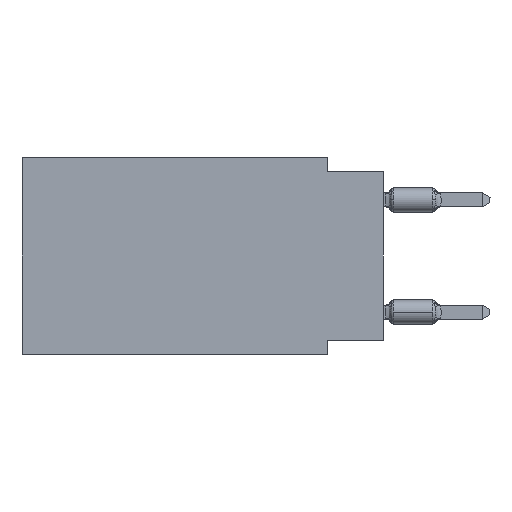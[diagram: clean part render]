
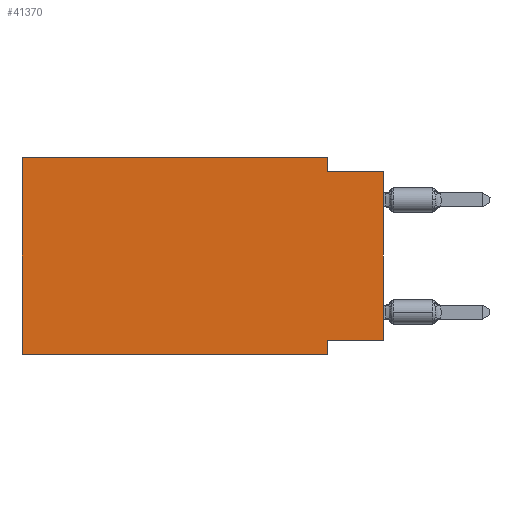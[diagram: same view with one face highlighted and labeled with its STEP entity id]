
A CAD part, left-side view. The second image highlights one B-rep face of the part: STEP entity #41370.
In plain terms, the highlighted planar face has unit normal (-1, 0, 0).
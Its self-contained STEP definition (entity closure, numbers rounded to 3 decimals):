
#964 = CARTESIAN_POINT ( 'NONE',  ( 0., 2.54, -8.255 ) ) ;
#1462 = VERTEX_POINT ( 'NONE', #51101 ) ;
#3433 = LINE ( 'NONE', #6978, #8571 ) ;
#3830 = CARTESIAN_POINT ( 'NONE',  ( 0., 0., -8.255 ) ) ;
#4790 = DIRECTION ( 'NONE',  ( 0., 1., 0. ) ) ;
#4881 = DIRECTION ( 'NONE',  ( 0., -1., 0. ) ) ;
#5058 = ORIENTED_EDGE ( 'NONE', *, *, #28933, .F. ) ;
#5126 = VERTEX_POINT ( 'NONE', #36732 ) ;
#6149 = ORIENTED_EDGE ( 'NONE', *, *, #12873, .F. ) ;
#6221 = VERTEX_POINT ( 'NONE', #964 ) ;
#6832 = LINE ( 'NONE', #12421, #51995 ) ;
#6978 = CARTESIAN_POINT ( 'NONE',  ( 0., 0., 0. ) ) ;
#8313 = ORIENTED_EDGE ( 'NONE', *, *, #32410, .F. ) ;
#8571 = VECTOR ( 'NONE', #29711, 1000. ) ;
#8636 = LINE ( 'NONE', #22224, #13220 ) ;
#10278 = ORIENTED_EDGE ( 'NONE', *, *, #24271, .F. ) ;
#12421 = CARTESIAN_POINT ( 'NONE',  ( 0., 16.383, 0. ) ) ;
#12873 = EDGE_CURVE ( 'NONE', #49265, #46509, #6832, .T. ) ;
#13220 = VECTOR ( 'NONE', #17785, 1000. ) ;
#15198 = VERTEX_POINT ( 'NONE', #29919 ) ;
#15246 = CARTESIAN_POINT ( 'NONE',  ( 0., 16.383, 0. ) ) ;
#15680 = DIRECTION ( 'NONE',  ( 0., -1., 0. ) ) ;
#17232 = CARTESIAN_POINT ( 'NONE',  ( 0., 0., -0.635 ) ) ;
#17785 = DIRECTION ( 'NONE',  ( 0., 0., -1. ) ) ;
#17814 = LINE ( 'NONE', #17232, #22514 ) ;
#18675 = VECTOR ( 'NONE', #36167, 1000. ) ;
#19339 = EDGE_CURVE ( 'NONE', #30919, #15198, #17814, .T. ) ;
#20586 = VECTOR ( 'NONE', #4790, 1000. ) ;
#20901 = CARTESIAN_POINT ( 'NONE',  ( 0., 2.54, -0.635 ) ) ;
#21305 = CARTESIAN_POINT ( 'NONE',  ( 0., 16.383, 0. ) ) ;
#22190 = VERTEX_POINT ( 'NONE', #3830 ) ;
#22216 = CARTESIAN_POINT ( 'NONE',  ( 0., 0., -8.255 ) ) ;
#22224 = CARTESIAN_POINT ( 'NONE',  ( 0., 2.54, 0. ) ) ;
#22330 = LINE ( 'NONE', #26758, #18675 ) ;
#22514 = VECTOR ( 'NONE', #36088, 1000. ) ;
#23429 = EDGE_LOOP ( 'NONE', ( #50246, #26756, #53212, #6149, #8313, #53117, #10278, #5058 ) ) ;
#24118 = DIRECTION ( 'NONE',  ( 0., 0., 1. ) ) ;
#24271 = EDGE_CURVE ( 'NONE', #6221, #1462, #22330, .T. ) ;
#24870 = FACE_OUTER_BOUND ( 'NONE', #23429, .T. ) ;
#26756 = ORIENTED_EDGE ( 'NONE', *, *, #19339, .F. ) ;
#26758 = CARTESIAN_POINT ( 'NONE',  ( 0., 2.54, -8.89 ) ) ;
#27256 = EDGE_CURVE ( 'NONE', #22190, #15198, #3433, .T. ) ;
#28550 = LINE ( 'NONE', #15246, #55770 ) ;
#28933 = EDGE_CURVE ( 'NONE', #22190, #6221, #45191, .T. ) ;
#29711 = DIRECTION ( 'NONE',  ( 0., 0., 1. ) ) ;
#29919 = CARTESIAN_POINT ( 'NONE',  ( 0., 0., -0.635 ) ) ;
#30088 = AXIS2_PLACEMENT_3D ( 'NONE', #21305, #56443, #35165 ) ;
#30919 = VERTEX_POINT ( 'NONE', #20901 ) ;
#32410 = EDGE_CURVE ( 'NONE', #5126, #49265, #28550, .T. ) ;
#35165 = DIRECTION ( 'NONE',  ( 0., 0., -1. ) ) ;
#36088 = DIRECTION ( 'NONE',  ( 0., -1., 0. ) ) ;
#36167 = DIRECTION ( 'NONE',  ( 0., 0., -1. ) ) ;
#36577 = CARTESIAN_POINT ( 'NONE',  ( 0., 16.383, 0. ) ) ;
#36732 = CARTESIAN_POINT ( 'NONE',  ( 0., 16.383, -8.89 ) ) ;
#37764 = VECTOR ( 'NONE', #4881, 1000. ) ;
#41370 = ADVANCED_FACE ( 'NONE', ( #24870 ), #43435, .F. ) ;
#43435 = PLANE ( 'NONE',  #30088 ) ;
#45191 = LINE ( 'NONE', #22216, #20586 ) ;
#45279 = CARTESIAN_POINT ( 'NONE',  ( 0., 16.383, -8.89 ) ) ;
#46509 = VERTEX_POINT ( 'NONE', #57489 ) ;
#46921 = EDGE_CURVE ( 'NONE', #46509, #30919, #8636, .T. ) ;
#48131 = EDGE_CURVE ( 'NONE', #5126, #1462, #54154, .T. ) ;
#49265 = VERTEX_POINT ( 'NONE', #36577 ) ;
#50246 = ORIENTED_EDGE ( 'NONE', *, *, #27256, .T. ) ;
#51101 = CARTESIAN_POINT ( 'NONE',  ( 0., 2.54, -8.89 ) ) ;
#51995 = VECTOR ( 'NONE', #15680, 1000. ) ;
#53117 = ORIENTED_EDGE ( 'NONE', *, *, #48131, .T. ) ;
#53212 = ORIENTED_EDGE ( 'NONE', *, *, #46921, .F. ) ;
#54154 = LINE ( 'NONE', #45279, #37764 ) ;
#55770 = VECTOR ( 'NONE', #24118, 1000. ) ;
#56443 = DIRECTION ( 'NONE',  ( 1., 0., 0. ) ) ;
#57489 = CARTESIAN_POINT ( 'NONE',  ( 0., 2.54, 0. ) ) ;
